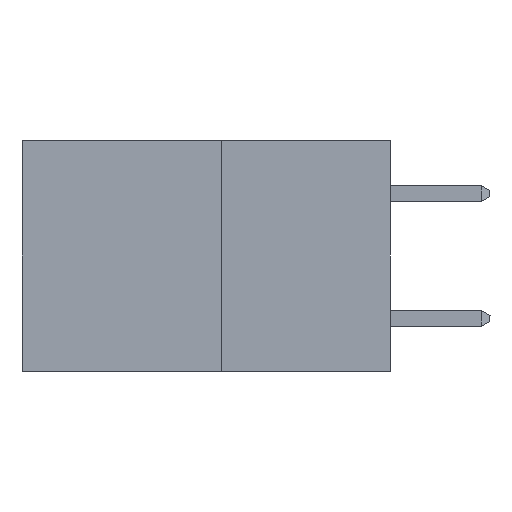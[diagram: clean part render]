
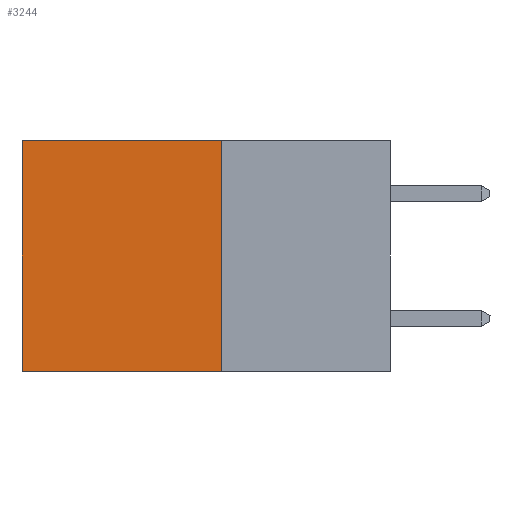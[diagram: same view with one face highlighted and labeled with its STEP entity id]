
A CAD part, left-side view. The second image highlights one B-rep face of the part: STEP entity #3244.
In plain terms, the highlighted planar face has unit normal (-1, 0, 0).
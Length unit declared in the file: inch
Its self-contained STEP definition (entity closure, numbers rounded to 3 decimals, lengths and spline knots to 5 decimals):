
#121 = VECTOR ( 'NONE', #7620, 39.37008 ) ;
#219 = ORIENTED_EDGE ( 'NONE', *, *, #2591, .F. ) ;
#232 = EDGE_CURVE ( 'NONE', #4174, #3745, #4240, .T. ) ;
#501 = ORIENTED_EDGE ( 'NONE', *, *, #2907, .T. ) ;
#784 = VECTOR ( 'NONE', #1952, 39.37008 ) ;
#1056 = LINE ( 'NONE', #3130, #784 ) ;
#1952 = DIRECTION ( 'NONE',  ( 0., 1., 0. ) ) ;
#2049 = DIRECTION ( 'NONE',  ( 0., 0., -1. ) ) ;
#2591 = EDGE_CURVE ( 'NONE', #3745, #7525, #1056, .T. ) ;
#2642 = CARTESIAN_POINT ( 'NONE',  ( 0.277, 0.59, -0.37 ) ) ;
#2907 = EDGE_CURVE ( 'NONE', #4174, #9378, #4441, .T. ) ;
#3130 = CARTESIAN_POINT ( 'NONE',  ( 0.277, 0.27, -0.37 ) ) ;
#3201 = AXIS2_PLACEMENT_3D ( 'NONE', #3753, #3618, #3752 ) ;
#3244 = ADVANCED_FACE ( 'NONE', ( #7671 ), #3804, .F. ) ;
#3253 = CARTESIAN_POINT ( 'NONE',  ( 0.277, 0.27, -0.37 ) ) ;
#3618 = DIRECTION ( 'NONE',  ( 1., 0., 0. ) ) ;
#3745 = VERTEX_POINT ( 'NONE', #5219 ) ;
#3752 = DIRECTION ( 'NONE',  ( 0., 0., -1. ) ) ;
#3753 = CARTESIAN_POINT ( 'NONE',  ( 0.277, 0.27, -0.37 ) ) ;
#3804 = PLANE ( 'NONE',  #3201 ) ;
#4174 = VERTEX_POINT ( 'NONE', #7809 ) ;
#4240 = LINE ( 'NONE', #3253, #10205 ) ;
#4441 = LINE ( 'NONE', #7634, #121 ) ;
#5219 = CARTESIAN_POINT ( 'NONE',  ( 0.277, 0.27, -0.37 ) ) ;
#5394 = CARTESIAN_POINT ( 'NONE',  ( 0.277, 0.59, 0. ) ) ;
#5594 = ORIENTED_EDGE ( 'NONE', *, *, #6544, .T. ) ;
#5776 = LINE ( 'NONE', #9186, #9827 ) ;
#6544 = EDGE_CURVE ( 'NONE', #9378, #7525, #5776, .T. ) ;
#6763 = ORIENTED_EDGE ( 'NONE', *, *, #232, .F. ) ;
#7525 = VERTEX_POINT ( 'NONE', #2642 ) ;
#7620 = DIRECTION ( 'NONE',  ( 0., 1., 0. ) ) ;
#7634 = CARTESIAN_POINT ( 'NONE',  ( 0.277, 0.27, 0. ) ) ;
#7671 = FACE_OUTER_BOUND ( 'NONE', #9080, .T. ) ;
#7809 = CARTESIAN_POINT ( 'NONE',  ( 0.277, 0.27, 0. ) ) ;
#9080 = EDGE_LOOP ( 'NONE', ( #5594, #219, #6763, #501 ) ) ;
#9145 = DIRECTION ( 'NONE',  ( 0., 0., -1. ) ) ;
#9186 = CARTESIAN_POINT ( 'NONE',  ( 0.277, 0.59, -0.37 ) ) ;
#9378 = VERTEX_POINT ( 'NONE', #5394 ) ;
#9827 = VECTOR ( 'NONE', #9145, 39.37008 ) ;
#10205 = VECTOR ( 'NONE', #2049, 39.37008 ) ;
